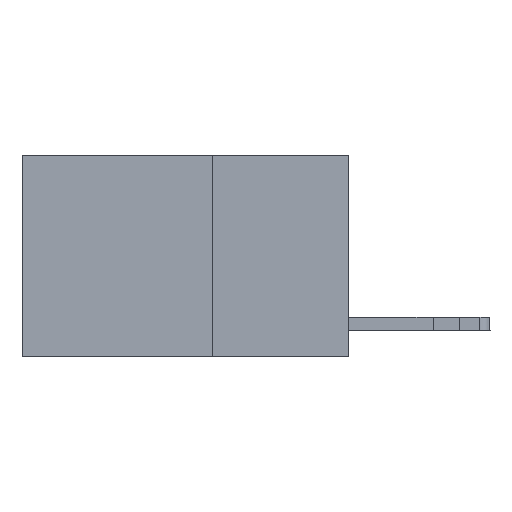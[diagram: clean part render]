
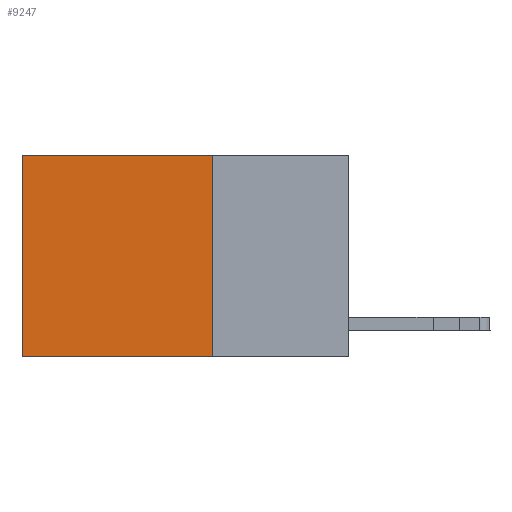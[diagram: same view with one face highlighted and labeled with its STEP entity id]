
A CAD part, left-side view. The second image highlights one B-rep face of the part: STEP entity #9247.
In plain terms, the highlighted planar face has unit normal (-1, 0, 0).
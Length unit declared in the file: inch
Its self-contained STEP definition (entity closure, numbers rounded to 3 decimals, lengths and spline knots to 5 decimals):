
#23 = VERTEX_POINT ( 'NONE', #6225 ) ;
#125 = LINE ( 'NONE', #12130, #5984 ) ;
#880 = EDGE_CURVE ( 'NONE', #23, #2592, #5875, .T. ) ;
#935 = VERTEX_POINT ( 'NONE', #5849 ) ;
#1062 = EDGE_LOOP ( 'NONE', ( #9994, #2562, #8770, #7193 ) ) ;
#1181 = PLANE ( 'NONE',  #2255 ) ;
#2255 = AXIS2_PLACEMENT_3D ( 'NONE', #4656, #12411, #5788 ) ;
#2359 = EDGE_CURVE ( 'NONE', #2592, #13462, #125, .T. ) ;
#2538 = LINE ( 'NONE', #3925, #8161 ) ;
#2562 = ORIENTED_EDGE ( 'NONE', *, *, #5785, .F. ) ;
#2592 = VERTEX_POINT ( 'NONE', #4846 ) ;
#2866 = VECTOR ( 'NONE', #5738, 39.37008 ) ;
#3925 = CARTESIAN_POINT ( 'NONE',  ( 0.2625, 0.25, -0.37 ) ) ;
#4656 = CARTESIAN_POINT ( 'NONE',  ( 0.2625, 0.25, 0. ) ) ;
#4812 = CARTESIAN_POINT ( 'NONE',  ( 0.2625, 0.25, 0. ) ) ;
#4846 = CARTESIAN_POINT ( 'NONE',  ( 0.2625, 0.6, 0. ) ) ;
#5738 = DIRECTION ( 'NONE',  ( 0., 1., 0. ) ) ;
#5785 = EDGE_CURVE ( 'NONE', #935, #13462, #2538, .T. ) ;
#5788 = DIRECTION ( 'NONE',  ( 0., 0., -1. ) ) ;
#5849 = CARTESIAN_POINT ( 'NONE',  ( 0.2625, 0.25, -0.37 ) ) ;
#5875 = LINE ( 'NONE', #10060, #2866 ) ;
#5963 = DIRECTION ( 'NONE',  ( 0., 0., -1. ) ) ;
#5984 = VECTOR ( 'NONE', #13212, 39.37008 ) ;
#6225 = CARTESIAN_POINT ( 'NONE',  ( 0.2625, 0.25, 0. ) ) ;
#7193 = ORIENTED_EDGE ( 'NONE', *, *, #880, .T. ) ;
#8161 = VECTOR ( 'NONE', #9358, 39.37008 ) ;
#8770 = ORIENTED_EDGE ( 'NONE', *, *, #10567, .F. ) ;
#9203 = FACE_OUTER_BOUND ( 'NONE', #1062, .T. ) ;
#9247 = ADVANCED_FACE ( 'NONE', ( #9203 ), #1181, .F. ) ;
#9358 = DIRECTION ( 'NONE',  ( 0., 1., 0. ) ) ;
#9582 = VECTOR ( 'NONE', #5963, 39.37008 ) ;
#9928 = LINE ( 'NONE', #4812, #9582 ) ;
#9994 = ORIENTED_EDGE ( 'NONE', *, *, #2359, .T. ) ;
#10060 = CARTESIAN_POINT ( 'NONE',  ( 0.2625, 0.25, 0. ) ) ;
#10567 = EDGE_CURVE ( 'NONE', #23, #935, #9928, .T. ) ;
#12130 = CARTESIAN_POINT ( 'NONE',  ( 0.2625, 0.6, 0. ) ) ;
#12411 = DIRECTION ( 'NONE',  ( 1., 0., 0. ) ) ;
#13212 = DIRECTION ( 'NONE',  ( 0., 0., -1. ) ) ;
#13392 = CARTESIAN_POINT ( 'NONE',  ( 0.2625, 0.6, -0.37 ) ) ;
#13462 = VERTEX_POINT ( 'NONE', #13392 ) ;
